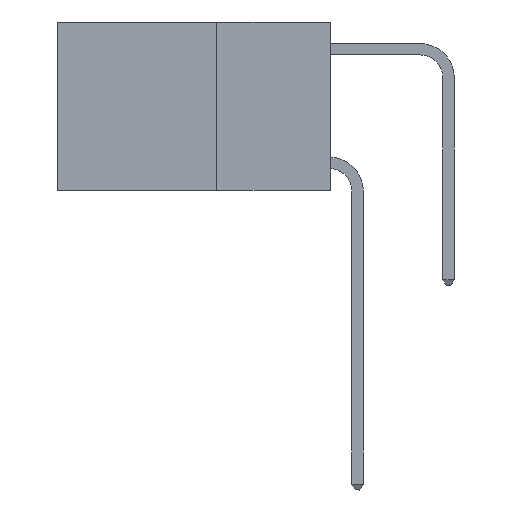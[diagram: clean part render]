
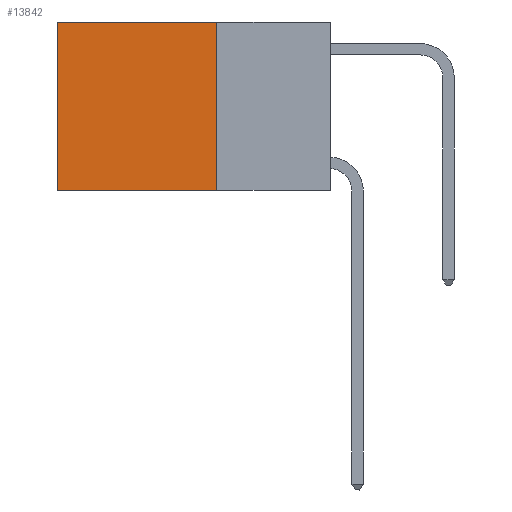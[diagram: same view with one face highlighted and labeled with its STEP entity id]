
A CAD part, left-side view. The second image highlights one B-rep face of the part: STEP entity #13842.
In plain terms, the highlighted planar face has unit normal (-1, 0, 0).
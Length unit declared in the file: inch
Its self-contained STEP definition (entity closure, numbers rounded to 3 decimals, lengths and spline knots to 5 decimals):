
#49 = PLANE ( 'NONE',  #11969 ) ;
#134 = CARTESIAN_POINT ( 'NONE',  ( 0.2625, 0.6, -0.37 ) ) ;
#776 = ORIENTED_EDGE ( 'NONE', *, *, #16846, .T. ) ;
#778 = VECTOR ( 'NONE', #1333, 39.37008 ) ;
#1329 = ORIENTED_EDGE ( 'NONE', *, *, #7338, .F. ) ;
#1333 = DIRECTION ( 'NONE',  ( 0., 1., 0. ) ) ;
#1789 = DIRECTION ( 'NONE',  ( 1., 0., 0. ) ) ;
#2382 = VERTEX_POINT ( 'NONE', #134 ) ;
#2717 = LINE ( 'NONE', #16845, #15757 ) ;
#4051 = CARTESIAN_POINT ( 'NONE',  ( 0.2625, 0.25, 0. ) ) ;
#4102 = EDGE_CURVE ( 'NONE', #5530, #2382, #14460, .T. ) ;
#5441 = LINE ( 'NONE', #4051, #18355 ) ;
#5466 = ORIENTED_EDGE ( 'NONE', *, *, #4102, .F. ) ;
#5530 = VERTEX_POINT ( 'NONE', #17361 ) ;
#5857 = DIRECTION ( 'NONE',  ( 0., 1., 0. ) ) ;
#5986 = ORIENTED_EDGE ( 'NONE', *, *, #7665, .T. ) ;
#6534 = LINE ( 'NONE', #20547, #14479 ) ;
#6583 = VERTEX_POINT ( 'NONE', #14763 ) ;
#7338 = EDGE_CURVE ( 'NONE', #16995, #5530, #2717, .T. ) ;
#7665 = EDGE_CURVE ( 'NONE', #16995, #6583, #5441, .T. ) ;
#8390 = DIRECTION ( 'NONE',  ( 0., 0., -1. ) ) ;
#9030 = FACE_OUTER_BOUND ( 'NONE', #15656, .T. ) ;
#9451 = CARTESIAN_POINT ( 'NONE',  ( 0.2625, 0.25, 0. ) ) ;
#11969 = AXIS2_PLACEMENT_3D ( 'NONE', #12063, #1789, #13773 ) ;
#12063 = CARTESIAN_POINT ( 'NONE',  ( 0.2625, 0.25, 0. ) ) ;
#13773 = DIRECTION ( 'NONE',  ( 0., 0., -1. ) ) ;
#13842 = ADVANCED_FACE ( 'NONE', ( #9030 ), #49, .F. ) ;
#14460 = LINE ( 'NONE', #21655, #778 ) ;
#14479 = VECTOR ( 'NONE', #17248, 39.37008 ) ;
#14763 = CARTESIAN_POINT ( 'NONE',  ( 0.2625, 0.6, 0. ) ) ;
#15656 = EDGE_LOOP ( 'NONE', ( #776, #5466, #1329, #5986 ) ) ;
#15757 = VECTOR ( 'NONE', #8390, 39.37008 ) ;
#16845 = CARTESIAN_POINT ( 'NONE',  ( 0.2625, 0.25, 0. ) ) ;
#16846 = EDGE_CURVE ( 'NONE', #6583, #2382, #6534, .T. ) ;
#16995 = VERTEX_POINT ( 'NONE', #9451 ) ;
#17248 = DIRECTION ( 'NONE',  ( 0., 0., -1. ) ) ;
#17361 = CARTESIAN_POINT ( 'NONE',  ( 0.2625, 0.25, -0.37 ) ) ;
#18355 = VECTOR ( 'NONE', #5857, 39.37008 ) ;
#20547 = CARTESIAN_POINT ( 'NONE',  ( 0.2625, 0.6, 0. ) ) ;
#21655 = CARTESIAN_POINT ( 'NONE',  ( 0.2625, 0.25, -0.37 ) ) ;
